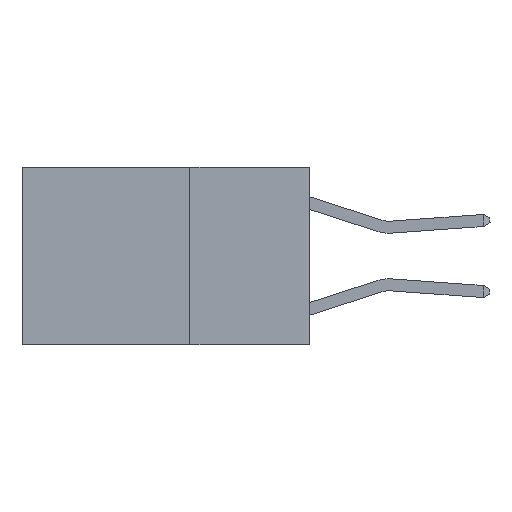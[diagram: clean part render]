
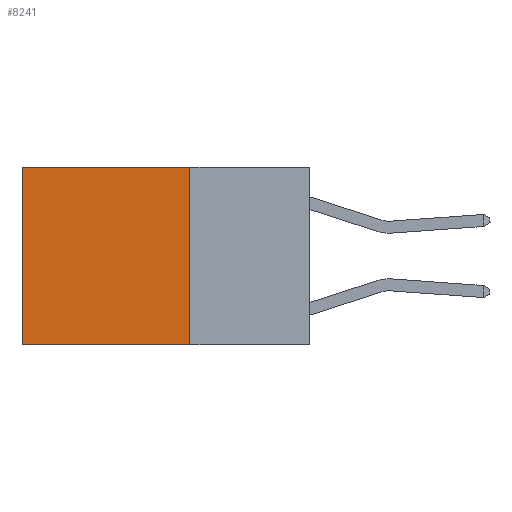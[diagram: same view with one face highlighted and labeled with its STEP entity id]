
A CAD part, left-side view. The second image highlights one B-rep face of the part: STEP entity #8241.
In plain terms, the highlighted planar face has unit normal (-1, 0, 0).
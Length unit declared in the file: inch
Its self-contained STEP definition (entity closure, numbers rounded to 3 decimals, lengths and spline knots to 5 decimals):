
#367 = LINE ( 'NONE', #8124, #1113 ) ;
#394 = ORIENTED_EDGE ( 'NONE', *, *, #10373, .T. ) ;
#576 = DIRECTION ( 'NONE',  ( 0., 1., 0. ) ) ;
#801 = EDGE_CURVE ( 'NONE', #13780, #2057, #10789, .T. ) ;
#922 = LINE ( 'NONE', #11747, #9798 ) ;
#1113 = VECTOR ( 'NONE', #576, 39.37008 ) ;
#1299 = LINE ( 'NONE', #7837, #5237 ) ;
#2057 = VERTEX_POINT ( 'NONE', #8360 ) ;
#2123 = CARTESIAN_POINT ( 'NONE',  ( 0.2625, 0.25, 0. ) ) ;
#2634 = ORIENTED_EDGE ( 'NONE', *, *, #801, .F. ) ;
#3209 = PLANE ( 'NONE',  #9958 ) ;
#3625 = EDGE_CURVE ( 'NONE', #2057, #12458, #367, .T. ) ;
#3926 = EDGE_CURVE ( 'NONE', #12759, #12458, #1299, .T. ) ;
#4282 = DIRECTION ( 'NONE',  ( 0., 1., 0. ) ) ;
#4717 = CARTESIAN_POINT ( 'NONE',  ( 0.2625, 0.25, 0. ) ) ;
#5237 = VECTOR ( 'NONE', #5535, 39.37008 ) ;
#5535 = DIRECTION ( 'NONE',  ( 0., 0., -1. ) ) ;
#6121 = ORIENTED_EDGE ( 'NONE', *, *, #3926, .T. ) ;
#6578 = DIRECTION ( 'NONE',  ( 0., 0., -1. ) ) ;
#7446 = EDGE_LOOP ( 'NONE', ( #6121, #11520, #2634, #394 ) ) ;
#7837 = CARTESIAN_POINT ( 'NONE',  ( 0.2625, 0.6, 0. ) ) ;
#8124 = CARTESIAN_POINT ( 'NONE',  ( 0.2625, 0.25, -0.37 ) ) ;
#8241 = ADVANCED_FACE ( 'NONE', ( #10817 ), #3209, .F. ) ;
#8360 = CARTESIAN_POINT ( 'NONE',  ( 0.2625, 0.25, -0.37 ) ) ;
#8722 = DIRECTION ( 'NONE',  ( 0., 0., -1. ) ) ;
#9798 = VECTOR ( 'NONE', #4282, 39.37008 ) ;
#9869 = CARTESIAN_POINT ( 'NONE',  ( 0.2625, 0.25, 0. ) ) ;
#9958 = AXIS2_PLACEMENT_3D ( 'NONE', #2123, #12970, #6578 ) ;
#10373 = EDGE_CURVE ( 'NONE', #13780, #12759, #922, .T. ) ;
#10789 = LINE ( 'NONE', #9869, #13331 ) ;
#10817 = FACE_OUTER_BOUND ( 'NONE', #7446, .T. ) ;
#11206 = CARTESIAN_POINT ( 'NONE',  ( 0.2625, 0.6, 0. ) ) ;
#11520 = ORIENTED_EDGE ( 'NONE', *, *, #3625, .F. ) ;
#11747 = CARTESIAN_POINT ( 'NONE',  ( 0.2625, 0.25, 0. ) ) ;
#12458 = VERTEX_POINT ( 'NONE', #13469 ) ;
#12759 = VERTEX_POINT ( 'NONE', #11206 ) ;
#12970 = DIRECTION ( 'NONE',  ( 1., 0., 0. ) ) ;
#13331 = VECTOR ( 'NONE', #8722, 39.37008 ) ;
#13469 = CARTESIAN_POINT ( 'NONE',  ( 0.2625, 0.6, -0.37 ) ) ;
#13780 = VERTEX_POINT ( 'NONE', #4717 ) ;
